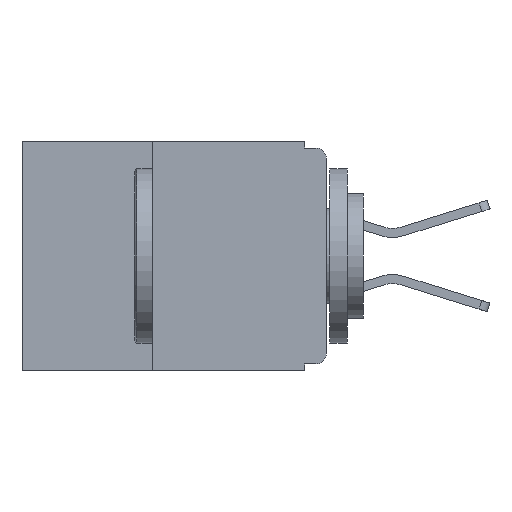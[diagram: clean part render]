
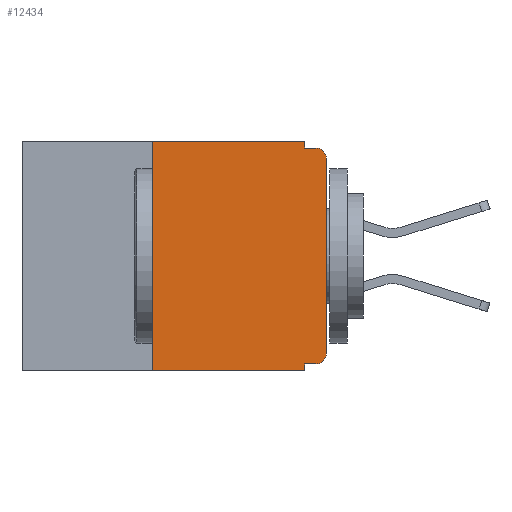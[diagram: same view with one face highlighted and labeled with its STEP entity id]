
A CAD part, left-side view. The second image highlights one B-rep face of the part: STEP entity #12434.
In plain terms, the highlighted planar face has unit normal (-1, 0, 0).
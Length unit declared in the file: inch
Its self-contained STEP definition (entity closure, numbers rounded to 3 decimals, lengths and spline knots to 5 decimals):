
#103 = ORIENTED_EDGE ( 'NONE', *, *, #22580, .F. ) ;
#459 = CARTESIAN_POINT ( 'NONE',  ( 0., 0.031, -0.33 ) ) ;
#952 = VERTEX_POINT ( 'NONE', #18609 ) ;
#1098 = CARTESIAN_POINT ( 'NONE',  ( 0., 0.437, 0. ) ) ;
#1864 = EDGE_CURVE ( 'NONE', #22791, #20685, #16395, .T. ) ;
#2227 = VECTOR ( 'NONE', #14993, 39.37008 ) ;
#3074 = VECTOR ( 'NONE', #14507, 39.37008 ) ;
#3267 = CARTESIAN_POINT ( 'NONE',  ( 0., 0.031, 0. ) ) ;
#3640 = VECTOR ( 'NONE', #5421, 39.37008 ) ;
#4178 = LINE ( 'NONE', #19860, #13711 ) ;
#4318 = AXIS2_PLACEMENT_3D ( 'NONE', #12235, #8698, #21151 ) ;
#5075 = PLANE ( 'NONE',  #4318 ) ;
#5269 = CARTESIAN_POINT ( 'NONE',  ( 0., 0.015, -0.305 ) ) ;
#5421 = DIRECTION ( 'NONE',  ( 0., 0., 1. ) ) ;
#6313 = DIRECTION ( 'NONE',  ( 0., -1., 0. ) ) ;
#6455 = VERTEX_POINT ( 'NONE', #8922 ) ;
#6549 = EDGE_CURVE ( 'NONE', #12669, #13816, #17835, .T. ) ;
#6745 = CIRCLE ( 'NONE', #17404, 0.015 ) ;
#7085 = DIRECTION ( 'NONE',  ( 0., 0., -1. ) ) ;
#7185 = DIRECTION ( 'NONE',  ( 0., 0., -1. ) ) ;
#7799 = LINE ( 'NONE', #18033, #3074 ) ;
#7842 = CARTESIAN_POINT ( 'NONE',  ( 0., 0.25, 0. ) ) ;
#8380 = LINE ( 'NONE', #17895, #3640 ) ;
#8698 = DIRECTION ( 'NONE',  ( 1., 0., 0. ) ) ;
#8922 = CARTESIAN_POINT ( 'NONE',  ( 0., 0.031, -0.33 ) ) ;
#9258 = FACE_OUTER_BOUND ( 'NONE', #13759, .T. ) ;
#9703 = CARTESIAN_POINT ( 'NONE',  ( 0., 0.015, -0.025 ) ) ;
#10392 = ORIENTED_EDGE ( 'NONE', *, *, #13169, .T. ) ;
#11563 = DIRECTION ( 'NONE',  ( 0., 0., -1. ) ) ;
#11599 = ORIENTED_EDGE ( 'NONE', *, *, #22485, .T. ) ;
#11825 = ORIENTED_EDGE ( 'NONE', *, *, #19076, .F. ) ;
#11985 = EDGE_CURVE ( 'NONE', #20685, #6455, #17067, .T. ) ;
#12078 = VERTEX_POINT ( 'NONE', #7842 ) ;
#12235 = CARTESIAN_POINT ( 'NONE',  ( 0., 0.437, 0. ) ) ;
#12303 = CARTESIAN_POINT ( 'NONE',  ( 0., 0.015, -0.32 ) ) ;
#12360 = ORIENTED_EDGE ( 'NONE', *, *, #20280, .F. ) ;
#12380 = VECTOR ( 'NONE', #21816, 39.37008 ) ;
#12434 = ADVANCED_FACE ( 'NONE', ( #9258 ), #5075, .F. ) ;
#12553 = VERTEX_POINT ( 'NONE', #12630 ) ;
#12630 = CARTESIAN_POINT ( 'NONE',  ( 0., 0., -0.305 ) ) ;
#12669 = VERTEX_POINT ( 'NONE', #14699 ) ;
#12731 = ORIENTED_EDGE ( 'NONE', *, *, #13778, .T. ) ;
#12799 = VECTOR ( 'NONE', #6313, 39.37008 ) ;
#12940 = AXIS2_PLACEMENT_3D ( 'NONE', #9703, #22121, #11563 ) ;
#13094 = ORIENTED_EDGE ( 'NONE', *, *, #11985, .F. ) ;
#13158 = VECTOR ( 'NONE', #21103, 39.37008 ) ;
#13169 = EDGE_CURVE ( 'NONE', #13944, #6455, #4178, .T. ) ;
#13186 = CARTESIAN_POINT ( 'NONE',  ( 0., 0.25, -0.33 ) ) ;
#13411 = ORIENTED_EDGE ( 'NONE', *, *, #1864, .F. ) ;
#13465 = LINE ( 'NONE', #19502, #17585 ) ;
#13523 = ORIENTED_EDGE ( 'NONE', *, *, #17745, .T. ) ;
#13711 = VECTOR ( 'NONE', #21649, 39.37008 ) ;
#13759 = EDGE_LOOP ( 'NONE', ( #12731, #11599, #21863, #12360, #103, #11825, #10392, #13094, #13411, #13523 ) ) ;
#13778 = EDGE_CURVE ( 'NONE', #12553, #952, #7799, .T. ) ;
#13816 = VERTEX_POINT ( 'NONE', #18193 ) ;
#13944 = VERTEX_POINT ( 'NONE', #13186 ) ;
#14265 = VERTEX_POINT ( 'NONE', #3267 ) ;
#14451 = CIRCLE ( 'NONE', #12940, 0.015 ) ;
#14507 = DIRECTION ( 'NONE',  ( 0., 0., 1. ) ) ;
#14699 = CARTESIAN_POINT ( 'NONE',  ( 0., 0.031, -0.01 ) ) ;
#14993 = DIRECTION ( 'NONE',  ( 0., 1., 0. ) ) ;
#16395 = LINE ( 'NONE', #18681, #2227 ) ;
#17067 = LINE ( 'NONE', #459, #12380 ) ;
#17404 = AXIS2_PLACEMENT_3D ( 'NONE', #5269, #17743, #7085 ) ;
#17585 = VECTOR ( 'NONE', #7185, 39.37008 ) ;
#17743 = DIRECTION ( 'NONE',  ( -1., 0., 0. ) ) ;
#17745 = EDGE_CURVE ( 'NONE', #22791, #12553, #6745, .T. ) ;
#17835 = LINE ( 'NONE', #21145, #13158 ) ;
#17895 = CARTESIAN_POINT ( 'NONE',  ( 0., 0.25, -0.33 ) ) ;
#18033 = CARTESIAN_POINT ( 'NONE',  ( 0., 0., 0. ) ) ;
#18193 = CARTESIAN_POINT ( 'NONE',  ( 0., 0.015, -0.01 ) ) ;
#18609 = CARTESIAN_POINT ( 'NONE',  ( 0., 0., -0.025 ) ) ;
#18681 = CARTESIAN_POINT ( 'NONE',  ( 0., 0., -0.32 ) ) ;
#19076 = EDGE_CURVE ( 'NONE', #13944, #12078, #8380, .T. ) ;
#19502 = CARTESIAN_POINT ( 'NONE',  ( 0., 0.031, 0. ) ) ;
#19860 = CARTESIAN_POINT ( 'NONE',  ( 0., 0.437, -0.33 ) ) ;
#20280 = EDGE_CURVE ( 'NONE', #14265, #12669, #13465, .T. ) ;
#20685 = VERTEX_POINT ( 'NONE', #22470 ) ;
#21103 = DIRECTION ( 'NONE',  ( 0., -1., 0. ) ) ;
#21145 = CARTESIAN_POINT ( 'NONE',  ( 0., 0., -0.01 ) ) ;
#21151 = DIRECTION ( 'NONE',  ( 0., 0., -1. ) ) ;
#21646 = LINE ( 'NONE', #1098, #12799 ) ;
#21649 = DIRECTION ( 'NONE',  ( 0., -1., 0. ) ) ;
#21816 = DIRECTION ( 'NONE',  ( 0., 0., -1. ) ) ;
#21863 = ORIENTED_EDGE ( 'NONE', *, *, #6549, .F. ) ;
#22121 = DIRECTION ( 'NONE',  ( -1., 0., 0. ) ) ;
#22470 = CARTESIAN_POINT ( 'NONE',  ( 0., 0.031, -0.32 ) ) ;
#22485 = EDGE_CURVE ( 'NONE', #952, #13816, #14451, .T. ) ;
#22580 = EDGE_CURVE ( 'NONE', #12078, #14265, #21646, .T. ) ;
#22791 = VERTEX_POINT ( 'NONE', #12303 ) ;
